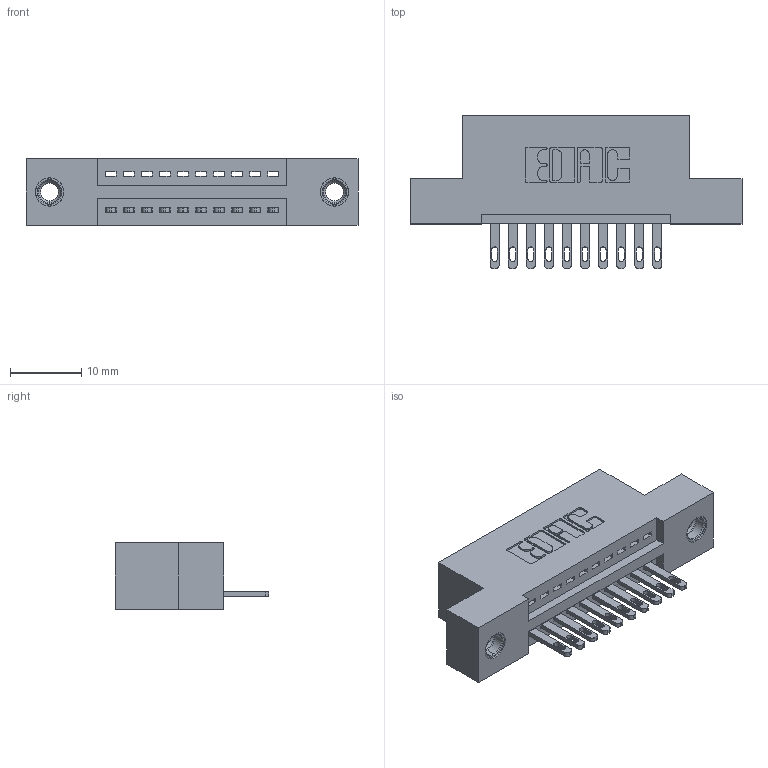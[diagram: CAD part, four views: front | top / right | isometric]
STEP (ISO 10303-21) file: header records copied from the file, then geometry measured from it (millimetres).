
FILE_DESCRIPTION (( 'STEP AP203' ), '1' );
FILE_NAME ('345-010-500-107.STEP', '2018-08-17T07:29:48', ( '' ), ( '' ), 'SwSTEP 2.0', 'SolidWorks 2016', '' );
FILE_SCHEMA (( 'CONFIG_CONTROL_DESIGN' ));
Length unit declared in the file: inch
Products named in the file (4): 345-010-500-107; 345 Part_Flush Mounting Lugs - 0.156 Dia-TI; 345-292-001_345-293-100; 345-250-001_345-250-005-103
Assembly tree (13 placements, depth 2):
  345-010-500-107
    345 Part_Flush Mounting Lugs - 0.156 Dia-TI
    345-292-001_345-293-100  x10
    345-250-001_345-250-005-103  x2
Bounding box: 46.61 x 21.51 x 9.4 mm (x, y, z)
Volume: 4157.5 mm3; surface area: 5145.1 mm2
Topology: 13 solids, 13 shells, 726 faces, 2157 edges, 1430 vertices
Faces by surface type: plane 452, cylinder 258, cone 12, torus 4
Entity records: 12950 total; most frequent: CARTESIAN_POINT 2225, ORIENTED_EDGE 2162, DIRECTION 2019, EDGE_CURVE 1081, LINE 885, VECTOR 885, VERTEX_POINT 716, AXIS2_PLACEMENT_3D 567
